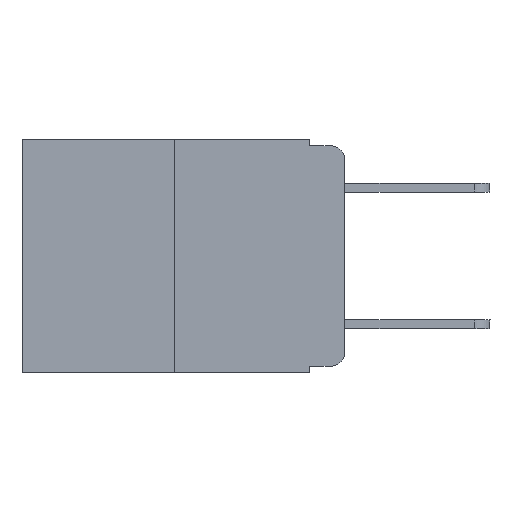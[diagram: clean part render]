
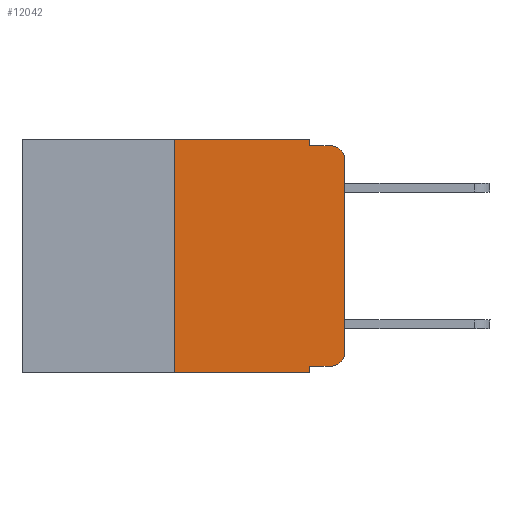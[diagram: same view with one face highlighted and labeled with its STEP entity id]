
A CAD part, left-side view. The second image highlights one B-rep face of the part: STEP entity #12042.
In plain terms, the highlighted planar face has unit normal (-1, 0, 0).
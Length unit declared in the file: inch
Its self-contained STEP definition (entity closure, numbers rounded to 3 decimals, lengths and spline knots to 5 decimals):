
#700 = DIRECTION ( 'NONE',  ( 0., -1., 0. ) ) ;
#747 = CARTESIAN_POINT ( 'NONE',  ( 0., 0., -0.03 ) ) ;
#858 = CARTESIAN_POINT ( 'NONE',  ( 0., 0.25, 0. ) ) ;
#1126 = LINE ( 'NONE', #858, #8078 ) ;
#1290 = VERTEX_POINT ( 'NONE', #3483 ) ;
#1393 = VERTEX_POINT ( 'NONE', #2395 ) ;
#1604 = CARTESIAN_POINT ( 'NONE',  ( 0., 0.25, 0. ) ) ;
#2143 = CARTESIAN_POINT ( 'NONE',  ( 0., 0.051, 0. ) ) ;
#2395 = CARTESIAN_POINT ( 'NONE',  ( 0., 0.02, -0.333 ) ) ;
#2693 = CARTESIAN_POINT ( 'NONE',  ( 0., 0.25, -0.343 ) ) ;
#3257 = DIRECTION ( 'NONE',  ( 1., 0., 0. ) ) ;
#3336 = CARTESIAN_POINT ( 'NONE',  ( 0., 0.051, -0.333 ) ) ;
#3483 = CARTESIAN_POINT ( 'NONE',  ( 0., 0.051, 0. ) ) ;
#3592 = LINE ( 'NONE', #3336, #15465 ) ;
#3671 = DIRECTION ( 'NONE',  ( -1., 0., 0. ) ) ;
#3787 = ORIENTED_EDGE ( 'NONE', *, *, #19647, .T. ) ;
#4841 = LINE ( 'NONE', #11341, #16334 ) ;
#5267 = EDGE_CURVE ( 'NONE', #20708, #7543, #24183, .T. ) ;
#5643 = FACE_OUTER_BOUND ( 'NONE', #24954, .T. ) ;
#5990 = DIRECTION ( 'NONE',  ( 0., 0., -1. ) ) ;
#6897 = LINE ( 'NONE', #22799, #22538 ) ;
#7268 = ORIENTED_EDGE ( 'NONE', *, *, #8728, .T. ) ;
#7543 = VERTEX_POINT ( 'NONE', #13774 ) ;
#7553 = CARTESIAN_POINT ( 'NONE',  ( 0., 0.02, -0.03 ) ) ;
#7564 = ORIENTED_EDGE ( 'NONE', *, *, #21894, .F. ) ;
#7664 = VECTOR ( 'NONE', #5990, 39.37008 ) ;
#8078 = VECTOR ( 'NONE', #20999, 39.37008 ) ;
#8211 = AXIS2_PLACEMENT_3D ( 'NONE', #7553, #3671, #15621 ) ;
#8696 = AXIS2_PLACEMENT_3D ( 'NONE', #12359, #14344, #14475 ) ;
#8728 = EDGE_CURVE ( 'NONE', #20708, #1393, #3592, .T. ) ;
#9506 = EDGE_CURVE ( 'NONE', #16212, #7543, #4841, .T. ) ;
#9909 = CARTESIAN_POINT ( 'NONE',  ( 0., 0.473, 0. ) ) ;
#9972 = CARTESIAN_POINT ( 'NONE',  ( 0., 0.02, -0.01 ) ) ;
#11178 = CIRCLE ( 'NONE', #8211, 0.02 ) ;
#11341 = CARTESIAN_POINT ( 'NONE',  ( 0., 0.473, -0.343 ) ) ;
#12042 = ADVANCED_FACE ( 'NONE', ( #5643 ), #19561, .F. ) ;
#12359 = CARTESIAN_POINT ( 'NONE',  ( 0., 0.02, -0.313 ) ) ;
#12746 = DIRECTION ( 'NONE',  ( 0., 0., 1. ) ) ;
#13085 = VERTEX_POINT ( 'NONE', #16590 ) ;
#13774 = CARTESIAN_POINT ( 'NONE',  ( 0., 0.051, -0.343 ) ) ;
#14138 = ORIENTED_EDGE ( 'NONE', *, *, #15492, .F. ) ;
#14344 = DIRECTION ( 'NONE',  ( -1., 0., 0. ) ) ;
#14403 = ORIENTED_EDGE ( 'NONE', *, *, #15811, .F. ) ;
#14475 = DIRECTION ( 'NONE',  ( 0., 0., -1. ) ) ;
#15086 = CARTESIAN_POINT ( 'NONE',  ( 0., 0.051, -0.01 ) ) ;
#15161 = VERTEX_POINT ( 'NONE', #15086 ) ;
#15457 = CARTESIAN_POINT ( 'NONE',  ( 0., 0.051, 0. ) ) ;
#15465 = VECTOR ( 'NONE', #26061, 39.37008 ) ;
#15492 = EDGE_CURVE ( 'NONE', #16212, #23689, #1126, .T. ) ;
#15592 = DIRECTION ( 'NONE',  ( 0., 0., -1. ) ) ;
#15605 = CARTESIAN_POINT ( 'NONE',  ( 0., 0.473, 0. ) ) ;
#15621 = DIRECTION ( 'NONE',  ( 0., 0., -1. ) ) ;
#15811 = EDGE_CURVE ( 'NONE', #23689, #1290, #23962, .T. ) ;
#16212 = VERTEX_POINT ( 'NONE', #2693 ) ;
#16334 = VECTOR ( 'NONE', #17435, 39.37008 ) ;
#16545 = VECTOR ( 'NONE', #17950, 39.37008 ) ;
#16590 = CARTESIAN_POINT ( 'NONE',  ( 0., 0., -0.313 ) ) ;
#16782 = VECTOR ( 'NONE', #15592, 39.37008 ) ;
#16830 = VERTEX_POINT ( 'NONE', #9972 ) ;
#16885 = CARTESIAN_POINT ( 'NONE',  ( 0., 0.051, -0.01 ) ) ;
#17435 = DIRECTION ( 'NONE',  ( 0., -1., 0. ) ) ;
#17705 = LINE ( 'NONE', #15457, #16782 ) ;
#17745 = ORIENTED_EDGE ( 'NONE', *, *, #21143, .T. ) ;
#17950 = DIRECTION ( 'NONE',  ( 0., -1., 0. ) ) ;
#18319 = VECTOR ( 'NONE', #700, 39.37008 ) ;
#18354 = ORIENTED_EDGE ( 'NONE', *, *, #9506, .T. ) ;
#18767 = VERTEX_POINT ( 'NONE', #747 ) ;
#18816 = ORIENTED_EDGE ( 'NONE', *, *, #5267, .F. ) ;
#19561 = PLANE ( 'NONE',  #20596 ) ;
#19647 = EDGE_CURVE ( 'NONE', #13085, #18767, #6897, .T. ) ;
#19679 = CIRCLE ( 'NONE', #8696, 0.02 ) ;
#19823 = DIRECTION ( 'NONE',  ( 0., 0., -1. ) ) ;
#20362 = ORIENTED_EDGE ( 'NONE', *, *, #25202, .F. ) ;
#20596 = AXIS2_PLACEMENT_3D ( 'NONE', #15605, #3257, #19823 ) ;
#20708 = VERTEX_POINT ( 'NONE', #23482 ) ;
#20999 = DIRECTION ( 'NONE',  ( 0., 0., 1. ) ) ;
#21143 = EDGE_CURVE ( 'NONE', #18767, #16830, #11178, .T. ) ;
#21894 = EDGE_CURVE ( 'NONE', #15161, #16830, #24754, .T. ) ;
#22538 = VECTOR ( 'NONE', #12746, 39.37008 ) ;
#22799 = CARTESIAN_POINT ( 'NONE',  ( 0., 0., 0. ) ) ;
#23482 = CARTESIAN_POINT ( 'NONE',  ( 0., 0.051, -0.333 ) ) ;
#23689 = VERTEX_POINT ( 'NONE', #1604 ) ;
#23962 = LINE ( 'NONE', #9909, #16545 ) ;
#24061 = EDGE_CURVE ( 'NONE', #1393, #13085, #19679, .T. ) ;
#24183 = LINE ( 'NONE', #2143, #7664 ) ;
#24597 = ORIENTED_EDGE ( 'NONE', *, *, #24061, .T. ) ;
#24754 = LINE ( 'NONE', #16885, #18319 ) ;
#24954 = EDGE_LOOP ( 'NONE', ( #3787, #17745, #7564, #20362, #14403, #14138, #18354, #18816, #7268, #24597 ) ) ;
#25202 = EDGE_CURVE ( 'NONE', #1290, #15161, #17705, .T. ) ;
#26061 = DIRECTION ( 'NONE',  ( 0., -1., 0. ) ) ;
